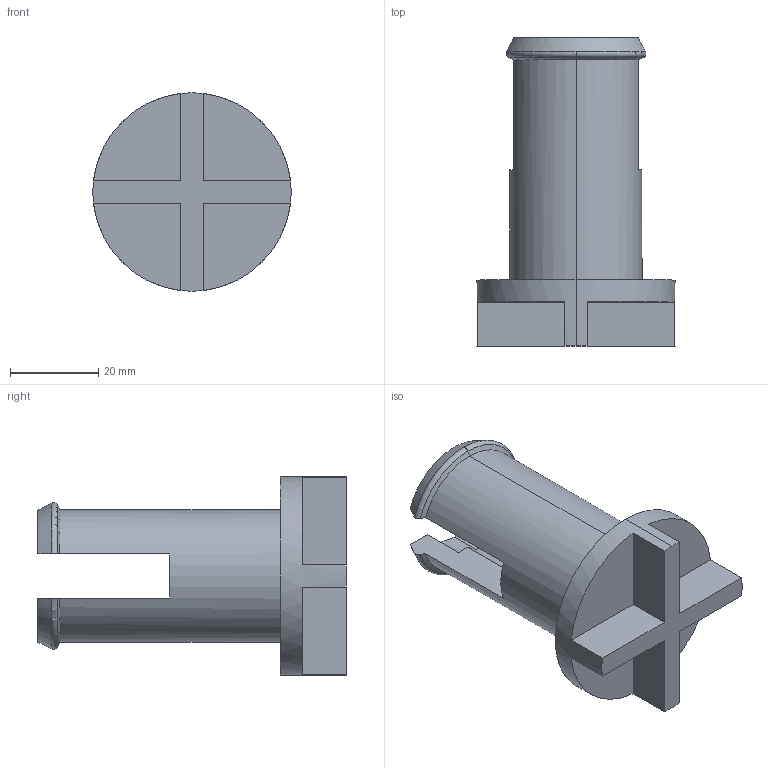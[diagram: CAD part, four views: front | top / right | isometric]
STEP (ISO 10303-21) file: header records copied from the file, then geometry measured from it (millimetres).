
FILE_DESCRIPTION (( 'STEP AP214' ), '1' );
FILE_NAME ('guide_rod.STEP', '2013-12-22T02:51:26', ( '' ), ( '' ), 'SwSTEP 2.0', 'SolidWorks 2013', '' );
FILE_SCHEMA (( 'AUTOMOTIVE_DESIGN' ));
Length unit declared in the file: millimetre
Products named in the file (1): guide_rod
Bounding box: 45 x 70 x 45 mm (x, y, z)
Volume: 35890.8 mm3; surface area: 13626.3 mm2
Topology: 1 solids, 1 shells, 47 faces, 130 edges, 86 vertices
Faces by surface type: plane 29, cylinder 9, cone 6, torus 3
Entity records: 1583 total; most frequent: CARTESIAN_POINT 320, DIRECTION 263, ORIENTED_EDGE 260, EDGE_CURVE 130, AXIS2_PLACEMENT_3D 97, VERTEX_POINT 86, LINE 69, VECTOR 69
